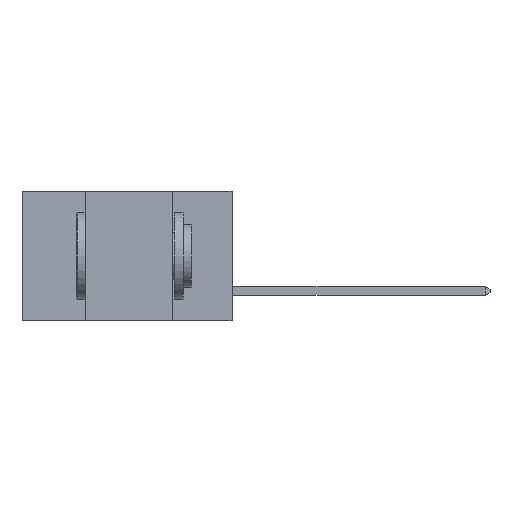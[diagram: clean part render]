
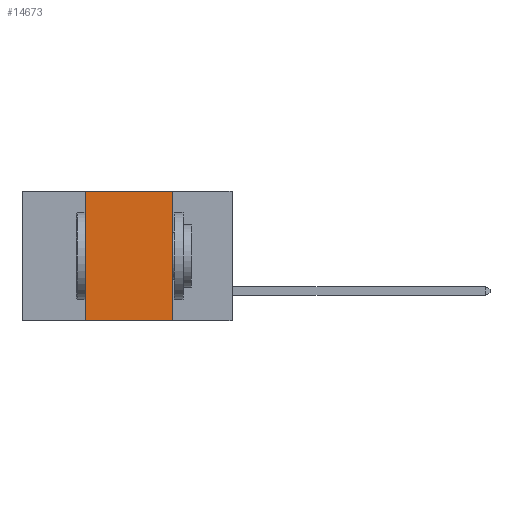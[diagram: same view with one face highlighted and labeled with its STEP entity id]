
A CAD part, left-side view. The second image highlights one B-rep face of the part: STEP entity #14673.
In plain terms, the highlighted planar face has unit normal (-1, 0, 0).
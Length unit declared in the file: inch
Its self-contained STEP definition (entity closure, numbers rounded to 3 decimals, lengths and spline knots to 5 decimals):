
#235 = VECTOR ( 'NONE', #13793, 39.37008 ) ;
#1395 = LINE ( 'NONE', #16143, #17843 ) ;
#3452 = LINE ( 'NONE', #7790, #11424 ) ;
#4286 = ORIENTED_EDGE ( 'NONE', *, *, #13800, .F. ) ;
#4442 = CARTESIAN_POINT ( 'NONE',  ( 0., 0.42, 0. ) ) ;
#4443 = LINE ( 'NONE', #18188, #12382 ) ;
#5271 = ORIENTED_EDGE ( 'NONE', *, *, #18310, .T. ) ;
#5909 = CARTESIAN_POINT ( 'NONE',  ( 0., 0.17, 0. ) ) ;
#7790 = CARTESIAN_POINT ( 'NONE',  ( 0., 0.17, 0. ) ) ;
#8435 = VERTEX_POINT ( 'NONE', #5909 ) ;
#8513 = ORIENTED_EDGE ( 'NONE', *, *, #17407, .F. ) ;
#9022 = LINE ( 'NONE', #12243, #235 ) ;
#9038 = AXIS2_PLACEMENT_3D ( 'NONE', #14100, #18779, #9448 ) ;
#9118 = VERTEX_POINT ( 'NONE', #20061 ) ;
#9448 = DIRECTION ( 'NONE',  ( 0., 0., -1. ) ) ;
#10952 = VERTEX_POINT ( 'NONE', #4442 ) ;
#11424 = VECTOR ( 'NONE', #18769, 39.37008 ) ;
#12243 = CARTESIAN_POINT ( 'NONE',  ( 0., 0.6, -0.37 ) ) ;
#12382 = VECTOR ( 'NONE', #19730, 39.37008 ) ;
#13340 = CARTESIAN_POINT ( 'NONE',  ( 0., 0.42, -0.37 ) ) ;
#13495 = VERTEX_POINT ( 'NONE', #13340 ) ;
#13793 = DIRECTION ( 'NONE',  ( 0., -1., 0. ) ) ;
#13800 = EDGE_CURVE ( 'NONE', #8435, #9118, #3452, .T. ) ;
#14100 = CARTESIAN_POINT ( 'NONE',  ( 0., 0.6, 0. ) ) ;
#14673 = ADVANCED_FACE ( 'NONE', ( #19159 ), #15672, .F. ) ;
#15672 = PLANE ( 'NONE',  #9038 ) ;
#16143 = CARTESIAN_POINT ( 'NONE',  ( 0., 0.6, 0. ) ) ;
#16222 = DIRECTION ( 'NONE',  ( 0., -1., 0. ) ) ;
#17310 = ORIENTED_EDGE ( 'NONE', *, *, #20159, .F. ) ;
#17407 = EDGE_CURVE ( 'NONE', #10952, #8435, #1395, .T. ) ;
#17843 = VECTOR ( 'NONE', #16222, 39.37008 ) ;
#17865 = EDGE_LOOP ( 'NONE', ( #4286, #8513, #17310, #5271 ) ) ;
#18188 = CARTESIAN_POINT ( 'NONE',  ( 0., 0.42, 0. ) ) ;
#18310 = EDGE_CURVE ( 'NONE', #13495, #9118, #9022, .T. ) ;
#18769 = DIRECTION ( 'NONE',  ( 0., 0., -1. ) ) ;
#18779 = DIRECTION ( 'NONE',  ( 1., 0., 0. ) ) ;
#19159 = FACE_OUTER_BOUND ( 'NONE', #17865, .T. ) ;
#19730 = DIRECTION ( 'NONE',  ( 0., 0., 1. ) ) ;
#20061 = CARTESIAN_POINT ( 'NONE',  ( 0., 0.17, -0.37 ) ) ;
#20159 = EDGE_CURVE ( 'NONE', #13495, #10952, #4443, .T. ) ;
